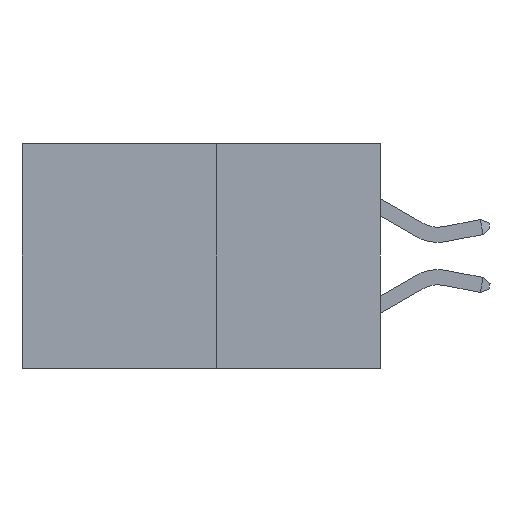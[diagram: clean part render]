
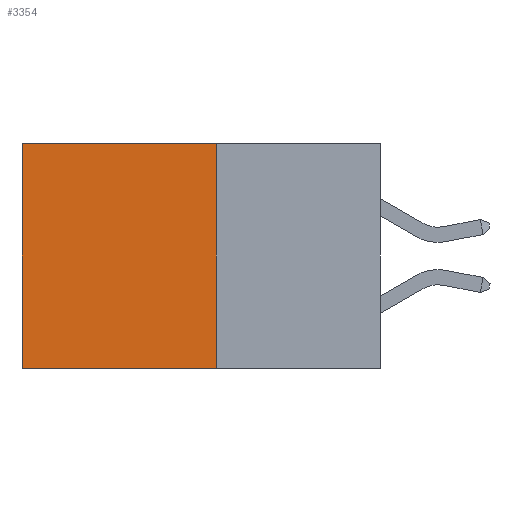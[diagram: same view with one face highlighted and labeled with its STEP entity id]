
A CAD part, left-side view. The second image highlights one B-rep face of the part: STEP entity #3354.
In plain terms, the highlighted planar face has unit normal (-1, 0, 0).
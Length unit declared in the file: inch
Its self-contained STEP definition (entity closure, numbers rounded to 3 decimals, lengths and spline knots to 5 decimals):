
#8 = DIRECTION ( 'NONE',  ( 1., 0., 0. ) ) ;
#649 = ORIENTED_EDGE ( 'NONE', *, *, #4899, .F. ) ;
#739 = ORIENTED_EDGE ( 'NONE', *, *, #2402, .F. ) ;
#846 = ORIENTED_EDGE ( 'NONE', *, *, #5701, .T. ) ;
#855 = DIRECTION ( 'NONE',  ( 0., 0., -1. ) ) ;
#882 = VECTOR ( 'NONE', #3239, 39.37008 ) ;
#1304 = VECTOR ( 'NONE', #7487, 39.37008 ) ;
#1494 = EDGE_LOOP ( 'NONE', ( #846, #649, #739, #2018 ) ) ;
#2018 = ORIENTED_EDGE ( 'NONE', *, *, #13309, .T. ) ;
#2274 = CARTESIAN_POINT ( 'NONE',  ( 0.277, 0.27, -0.37 ) ) ;
#2402 = EDGE_CURVE ( 'NONE', #4245, #9821, #14222, .T. ) ;
#2702 = LINE ( 'NONE', #13126, #8465 ) ;
#3239 = DIRECTION ( 'NONE',  ( 0., 1., 0. ) ) ;
#3354 = ADVANCED_FACE ( 'NONE', ( #9276 ), #14418, .F. ) ;
#4245 = VERTEX_POINT ( 'NONE', #4332 ) ;
#4332 = CARTESIAN_POINT ( 'NONE',  ( 0.277, 0.27, 0. ) ) ;
#4758 = VERTEX_POINT ( 'NONE', #8692 ) ;
#4899 = EDGE_CURVE ( 'NONE', #9821, #4758, #13051, .T. ) ;
#5701 = EDGE_CURVE ( 'NONE', #7384, #4758, #2702, .T. ) ;
#6193 = CARTESIAN_POINT ( 'NONE',  ( 0.277, 0.27, -0.37 ) ) ;
#6434 = CARTESIAN_POINT ( 'NONE',  ( 0.277, 0.27, 0. ) ) ;
#7181 = CARTESIAN_POINT ( 'NONE',  ( 0.277, 0.27, -0.37 ) ) ;
#7384 = VERTEX_POINT ( 'NONE', #11969 ) ;
#7487 = DIRECTION ( 'NONE',  ( 0., 1., 0. ) ) ;
#7642 = LINE ( 'NONE', #6434, #1304 ) ;
#8465 = VECTOR ( 'NONE', #12900, 39.37008 ) ;
#8692 = CARTESIAN_POINT ( 'NONE',  ( 0.277, 0.59, -0.37 ) ) ;
#8775 = DIRECTION ( 'NONE',  ( 0., 0., -1. ) ) ;
#9276 = FACE_OUTER_BOUND ( 'NONE', #1494, .T. ) ;
#9821 = VERTEX_POINT ( 'NONE', #7181 ) ;
#11969 = CARTESIAN_POINT ( 'NONE',  ( 0.277, 0.59, 0. ) ) ;
#12900 = DIRECTION ( 'NONE',  ( 0., 0., -1. ) ) ;
#13051 = LINE ( 'NONE', #2274, #882 ) ;
#13126 = CARTESIAN_POINT ( 'NONE',  ( 0.277, 0.59, -0.37 ) ) ;
#13309 = EDGE_CURVE ( 'NONE', #4245, #7384, #7642, .T. ) ;
#13362 = AXIS2_PLACEMENT_3D ( 'NONE', #14764, #8, #855 ) ;
#13878 = VECTOR ( 'NONE', #8775, 39.37008 ) ;
#14222 = LINE ( 'NONE', #6193, #13878 ) ;
#14418 = PLANE ( 'NONE',  #13362 ) ;
#14764 = CARTESIAN_POINT ( 'NONE',  ( 0.277, 0.27, -0.37 ) ) ;
